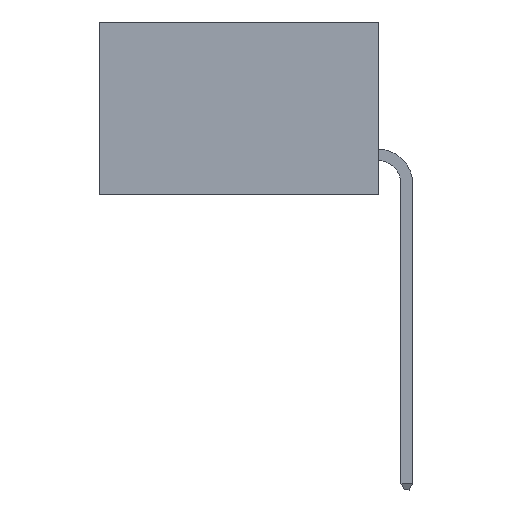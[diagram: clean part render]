
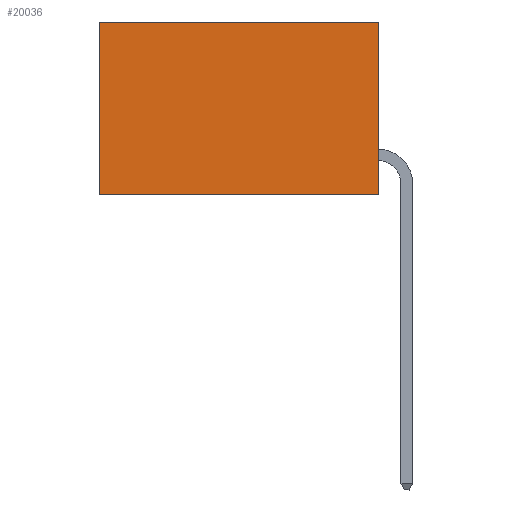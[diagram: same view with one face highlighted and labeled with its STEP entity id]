
A CAD part, left-side view. The second image highlights one B-rep face of the part: STEP entity #20036.
In plain terms, the highlighted planar face has unit normal (-1, 0, 0).
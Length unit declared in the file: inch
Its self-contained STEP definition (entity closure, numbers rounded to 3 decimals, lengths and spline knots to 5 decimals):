
#197 = DIRECTION ( 'NONE',  ( 0., 1., 0. ) ) ;
#673 = DIRECTION ( 'NONE',  ( 0., 0., -1. ) ) ;
#1096 = ORIENTED_EDGE ( 'NONE', *, *, #7176, .T. ) ;
#1857 = CARTESIAN_POINT ( 'NONE',  ( 0.2615, 0., -0.37 ) ) ;
#2172 = ORIENTED_EDGE ( 'NONE', *, *, #2648, .F. ) ;
#2648 = EDGE_CURVE ( 'NONE', #18515, #6239, #7113, .T. ) ;
#4133 = CARTESIAN_POINT ( 'NONE',  ( 0.2615, 0.6, -0.37 ) ) ;
#4422 = FACE_OUTER_BOUND ( 'NONE', #11903, .T. ) ;
#5101 = CARTESIAN_POINT ( 'NONE',  ( 0.2615, 0., -0.37 ) ) ;
#6160 = CARTESIAN_POINT ( 'NONE',  ( 0.2615, 0.6, -0.37 ) ) ;
#6239 = VERTEX_POINT ( 'NONE', #6160 ) ;
#6484 = DIRECTION ( 'NONE',  ( 0., 0., -1. ) ) ;
#6812 = EDGE_CURVE ( 'NONE', #21847, #18515, #15676, .T. ) ;
#7113 = LINE ( 'NONE', #1857, #10544 ) ;
#7176 = EDGE_CURVE ( 'NONE', #12916, #6239, #20126, .T. ) ;
#7865 = AXIS2_PLACEMENT_3D ( 'NONE', #16671, #22404, #673 ) ;
#9721 = PLANE ( 'NONE',  #7865 ) ;
#9774 = DIRECTION ( 'NONE',  ( 0., 1., 0. ) ) ;
#10464 = CARTESIAN_POINT ( 'NONE',  ( 0.2615, 0.6, 0. ) ) ;
#10544 = VECTOR ( 'NONE', #197, 39.37008 ) ;
#11431 = CARTESIAN_POINT ( 'NONE',  ( 0.2615, 0., 0. ) ) ;
#11744 = ORIENTED_EDGE ( 'NONE', *, *, #17896, .T. ) ;
#11903 = EDGE_LOOP ( 'NONE', ( #1096, #2172, #16159, #11744 ) ) ;
#11979 = VECTOR ( 'NONE', #16604, 39.37008 ) ;
#12032 = CARTESIAN_POINT ( 'NONE',  ( 0.2615, 0., -0.37 ) ) ;
#12680 = VECTOR ( 'NONE', #9774, 39.37008 ) ;
#12916 = VERTEX_POINT ( 'NONE', #10464 ) ;
#14762 = VECTOR ( 'NONE', #6484, 39.37008 ) ;
#15067 = LINE ( 'NONE', #11431, #12680 ) ;
#15676 = LINE ( 'NONE', #12032, #14762 ) ;
#16122 = CARTESIAN_POINT ( 'NONE',  ( 0.2615, 0., 0. ) ) ;
#16159 = ORIENTED_EDGE ( 'NONE', *, *, #6812, .F. ) ;
#16604 = DIRECTION ( 'NONE',  ( 0., 0., -1. ) ) ;
#16671 = CARTESIAN_POINT ( 'NONE',  ( 0.2615, 0., -0.37 ) ) ;
#17896 = EDGE_CURVE ( 'NONE', #21847, #12916, #15067, .T. ) ;
#18515 = VERTEX_POINT ( 'NONE', #5101 ) ;
#20036 = ADVANCED_FACE ( 'NONE', ( #4422 ), #9721, .F. ) ;
#20126 = LINE ( 'NONE', #4133, #11979 ) ;
#21847 = VERTEX_POINT ( 'NONE', #16122 ) ;
#22404 = DIRECTION ( 'NONE',  ( 1., 0., 0. ) ) ;
